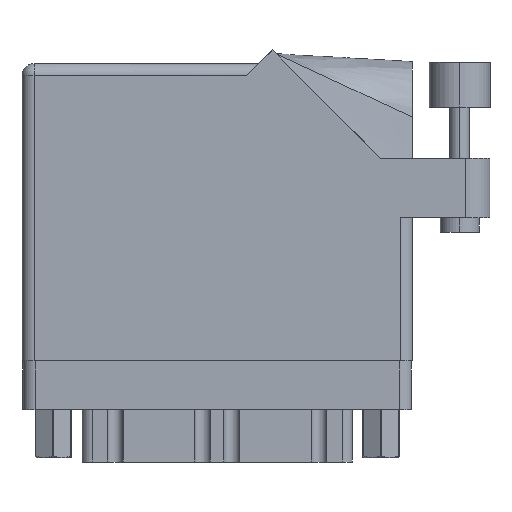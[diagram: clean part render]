
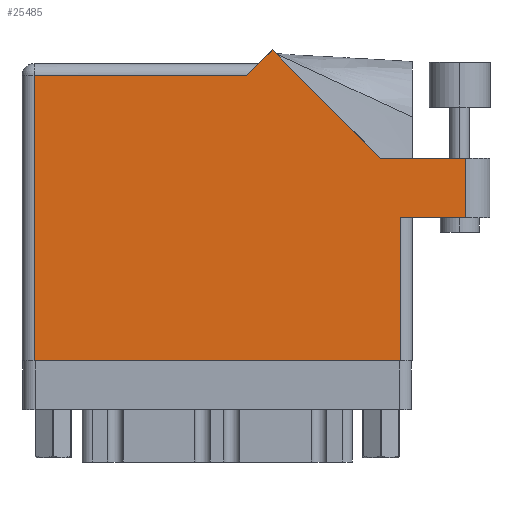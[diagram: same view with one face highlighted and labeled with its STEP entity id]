
A CAD part, front view. The second image highlights one B-rep face of the part: STEP entity #25485.
In plain terms, the highlighted face is planar.
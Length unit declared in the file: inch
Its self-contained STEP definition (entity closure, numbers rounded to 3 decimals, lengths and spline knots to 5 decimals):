
#393 = LINE ( 'NONE', #31289, #19459 ) ;
#601 = CARTESIAN_POINT ( 'NONE',  ( 0., 1.468, 0. ) ) ;
#981 = VERTEX_POINT ( 'NONE', #3478 ) ;
#1183 = EDGE_CURVE ( 'NONE', #27713, #25487, #38095, .T. ) ;
#1469 = CARTESIAN_POINT ( 'NONE',  ( 0., 1.53, 0. ) ) ;
#2556 = VERTEX_POINT ( 'NONE', #15834 ) ;
#3469 = ORIENTED_EDGE ( 'NONE', *, *, #21971, .T. ) ;
#3478 = CARTESIAN_POINT ( 'NONE',  ( 1.948, 0.737, 0. ) ) ;
#4769 = CARTESIAN_POINT ( 'NONE',  ( 0.062, 0., 0. ) ) ;
#5845 = ORIENTED_EDGE ( 'NONE', *, *, #25426, .T. ) ;
#6785 = CARTESIAN_POINT ( 'NONE',  ( 1.217, 1.53, 0. ) ) ;
#7576 = DIRECTION ( 'NONE',  ( 0., -1., 0. ) ) ;
#8016 = LINE ( 'NONE', #31390, #42655 ) ;
#10283 = VECTOR ( 'NONE', #25069, 39.37008 ) ;
#10529 = ORIENTED_EDGE ( 'NONE', *, *, #35606, .T. ) ;
#11117 = CARTESIAN_POINT ( 'NONE',  ( 2.285, 1.044, 0. ) ) ;
#11386 = DIRECTION ( 'NONE',  ( 0., 0., -1. ) ) ;
#11631 = CARTESIAN_POINT ( 'NONE',  ( 0., 0., 0. ) ) ;
#11665 = ORIENTED_EDGE ( 'NONE', *, *, #38300, .T. ) ;
#13859 = VERTEX_POINT ( 'NONE', #25841 ) ;
#14513 = DIRECTION ( 'NONE',  ( 1., 0., 0. ) ) ;
#14919 = DIRECTION ( 'NONE',  ( -1., 0., 0. ) ) ;
#15498 = VECTOR ( 'NONE', #20676, 39.37008 ) ;
#15682 = VERTEX_POINT ( 'NONE', #11117 ) ;
#15834 = CARTESIAN_POINT ( 'NONE',  ( 1.84442, 1.044, 0. ) ) ;
#16044 = VECTOR ( 'NONE', #19323, 39.37008 ) ;
#16737 = VECTOR ( 'NONE', #30799, 39.37008 ) ;
#16826 = VERTEX_POINT ( 'NONE', #21135 ) ;
#17008 = DIRECTION ( 'NONE',  ( -1., 0., 0. ) ) ;
#17591 = DIRECTION ( 'NONE',  ( -1., 0., 0. ) ) ;
#19323 = DIRECTION ( 'NONE',  ( -0.707, 0.707, 0. ) ) ;
#19459 = VECTOR ( 'NONE', #14513, 39.37008 ) ;
#20676 = DIRECTION ( 'NONE',  ( -0.707, -0.707, 0. ) ) ;
#20860 = CARTESIAN_POINT ( 'NONE',  ( 0.062, 1.468, 0. ) ) ;
#21135 = CARTESIAN_POINT ( 'NONE',  ( 1.948, 0., 0. ) ) ;
#21194 = LINE ( 'NONE', #31336, #40215 ) ;
#21392 = LINE ( 'NONE', #38158, #16044 ) ;
#21971 = EDGE_CURVE ( 'NONE', #15682, #2556, #21194, .T. ) ;
#22598 = LINE ( 'NONE', #25492, #34350 ) ;
#23752 = LINE ( 'NONE', #6785, #15498 ) ;
#24059 = VERTEX_POINT ( 'NONE', #4769 ) ;
#24377 = FACE_OUTER_BOUND ( 'NONE', #25344, .T. ) ;
#25069 = DIRECTION ( 'NONE',  ( 1., 0., 0. ) ) ;
#25344 = EDGE_LOOP ( 'NONE', ( #42146, #5845, #3469, #11665, #40144, #33150, #10529, #31478, #33314 ) ) ;
#25426 = EDGE_CURVE ( 'NONE', #27950, #15682, #34108, .T. ) ;
#25485 = ADVANCED_FACE ( 'NONE', ( #24377 ), #37624, .F. ) ;
#25487 = VERTEX_POINT ( 'NONE', #20860 ) ;
#25492 = CARTESIAN_POINT ( 'NONE',  ( 1.948, 0.737, 0. ) ) ;
#25841 = CARTESIAN_POINT ( 'NONE',  ( 1.28771, 1.60071, 0. ) ) ;
#26918 = EDGE_CURVE ( 'NONE', #16826, #981, #22598, .T. ) ;
#27418 = CARTESIAN_POINT ( 'NONE',  ( 1.155, 1.468, 0. ) ) ;
#27713 = VERTEX_POINT ( 'NONE', #27418 ) ;
#27950 = VERTEX_POINT ( 'NONE', #42828 ) ;
#29358 = EDGE_CURVE ( 'NONE', #981, #27950, #393, .T. ) ;
#30799 = DIRECTION ( 'NONE',  ( 0., 1., 0. ) ) ;
#31289 = CARTESIAN_POINT ( 'NONE',  ( 2.01, 0.737, 0. ) ) ;
#31336 = CARTESIAN_POINT ( 'NONE',  ( 2.41, 1.044, 0. ) ) ;
#31390 = CARTESIAN_POINT ( 'NONE',  ( 0.062, 0., 0. ) ) ;
#31478 = ORIENTED_EDGE ( 'NONE', *, *, #43244, .T. ) ;
#33150 = ORIENTED_EDGE ( 'NONE', *, *, #1183, .T. ) ;
#33314 = ORIENTED_EDGE ( 'NONE', *, *, #26918, .T. ) ;
#33648 = AXIS2_PLACEMENT_3D ( 'NONE', #1469, #11386, #14919 ) ;
#34108 = LINE ( 'NONE', #34772, #16737 ) ;
#34350 = VECTOR ( 'NONE', #38747, 39.37008 ) ;
#34772 = CARTESIAN_POINT ( 'NONE',  ( 2.285, 1.044, 0. ) ) ;
#35606 = EDGE_CURVE ( 'NONE', #25487, #24059, #8016, .T. ) ;
#36129 = VECTOR ( 'NONE', #17591, 39.37008 ) ;
#37624 = PLANE ( 'NONE',  #33648 ) ;
#38095 = LINE ( 'NONE', #601, #36129 ) ;
#38158 = CARTESIAN_POINT ( 'NONE',  ( 1.84442, 1.044, 0. ) ) ;
#38300 = EDGE_CURVE ( 'NONE', #2556, #13859, #21392, .T. ) ;
#38747 = DIRECTION ( 'NONE',  ( 0., 1., 0. ) ) ;
#40144 = ORIENTED_EDGE ( 'NONE', *, *, #40628, .T. ) ;
#40215 = VECTOR ( 'NONE', #17008, 39.37008 ) ;
#40628 = EDGE_CURVE ( 'NONE', #13859, #27713, #23752, .T. ) ;
#41863 = LINE ( 'NONE', #11631, #10283 ) ;
#42146 = ORIENTED_EDGE ( 'NONE', *, *, #29358, .T. ) ;
#42655 = VECTOR ( 'NONE', #7576, 39.37008 ) ;
#42828 = CARTESIAN_POINT ( 'NONE',  ( 2.285, 0.737, 0. ) ) ;
#43244 = EDGE_CURVE ( 'NONE', #24059, #16826, #41863, .T. ) ;
